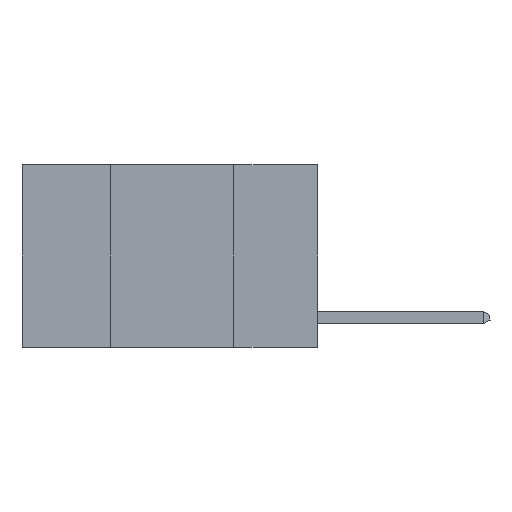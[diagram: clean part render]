
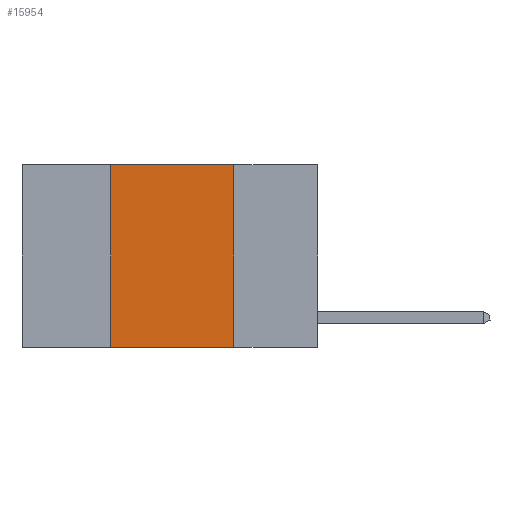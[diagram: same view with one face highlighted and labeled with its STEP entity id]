
A CAD part, left-side view. The second image highlights one B-rep face of the part: STEP entity #15954.
In plain terms, the highlighted planar face has unit normal (-1, 0, 0).
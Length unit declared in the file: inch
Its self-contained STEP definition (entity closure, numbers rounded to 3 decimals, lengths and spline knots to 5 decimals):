
#24 = CARTESIAN_POINT ( 'NONE',  ( 0., 0.6, -0.37 ) ) ;
#118 = LINE ( 'NONE', #3252, #12349 ) ;
#530 = LINE ( 'NONE', #24, #4806 ) ;
#844 = ORIENTED_EDGE ( 'NONE', *, *, #16485, .F. ) ;
#1568 = PLANE ( 'NONE',  #13850 ) ;
#1837 = VECTOR ( 'NONE', #2332, 39.37008 ) ;
#2332 = DIRECTION ( 'NONE',  ( 0., -1., 0. ) ) ;
#3196 = DIRECTION ( 'NONE',  ( 0., 0., -1. ) ) ;
#3252 = CARTESIAN_POINT ( 'NONE',  ( 0., 0.42, 0. ) ) ;
#3909 = FACE_OUTER_BOUND ( 'NONE', #9121, .T. ) ;
#4806 = VECTOR ( 'NONE', #14345, 39.37008 ) ;
#4844 = DIRECTION ( 'NONE',  ( 0., 0., 1. ) ) ;
#5318 = EDGE_CURVE ( 'NONE', #20404, #6909, #118, .T. ) ;
#6586 = LINE ( 'NONE', #15076, #1837 ) ;
#6622 = VECTOR ( 'NONE', #10732, 39.37008 ) ;
#6726 = EDGE_CURVE ( 'NONE', #6909, #18988, #6586, .T. ) ;
#6909 = VERTEX_POINT ( 'NONE', #17077 ) ;
#7798 = CARTESIAN_POINT ( 'NONE',  ( 0., 0.42, -0.37 ) ) ;
#9121 = EDGE_LOOP ( 'NONE', ( #844, #9327, #18304, #14571 ) ) ;
#9129 = CARTESIAN_POINT ( 'NONE',  ( 0., 0.17, 0. ) ) ;
#9327 = ORIENTED_EDGE ( 'NONE', *, *, #6726, .F. ) ;
#9888 = VERTEX_POINT ( 'NONE', #16633 ) ;
#10732 = DIRECTION ( 'NONE',  ( 0., 0., -1. ) ) ;
#12349 = VECTOR ( 'NONE', #4844, 39.37008 ) ;
#12699 = DIRECTION ( 'NONE',  ( 1., 0., 0. ) ) ;
#13850 = AXIS2_PLACEMENT_3D ( 'NONE', #19011, #12699, #3196 ) ;
#14345 = DIRECTION ( 'NONE',  ( 0., -1., 0. ) ) ;
#14571 = ORIENTED_EDGE ( 'NONE', *, *, #18622, .T. ) ;
#14580 = LINE ( 'NONE', #9129, #6622 ) ;
#15076 = CARTESIAN_POINT ( 'NONE',  ( 0., 0.6, 0. ) ) ;
#15954 = ADVANCED_FACE ( 'NONE', ( #3909 ), #1568, .F. ) ;
#16485 = EDGE_CURVE ( 'NONE', #18988, #9888, #14580, .T. ) ;
#16633 = CARTESIAN_POINT ( 'NONE',  ( 0., 0.17, -0.37 ) ) ;
#17077 = CARTESIAN_POINT ( 'NONE',  ( 0., 0.42, 0. ) ) ;
#18304 = ORIENTED_EDGE ( 'NONE', *, *, #5318, .F. ) ;
#18622 = EDGE_CURVE ( 'NONE', #20404, #9888, #530, .T. ) ;
#18988 = VERTEX_POINT ( 'NONE', #19983 ) ;
#19011 = CARTESIAN_POINT ( 'NONE',  ( 0., 0.6, 0. ) ) ;
#19983 = CARTESIAN_POINT ( 'NONE',  ( 0., 0.17, 0. ) ) ;
#20404 = VERTEX_POINT ( 'NONE', #7798 ) ;
